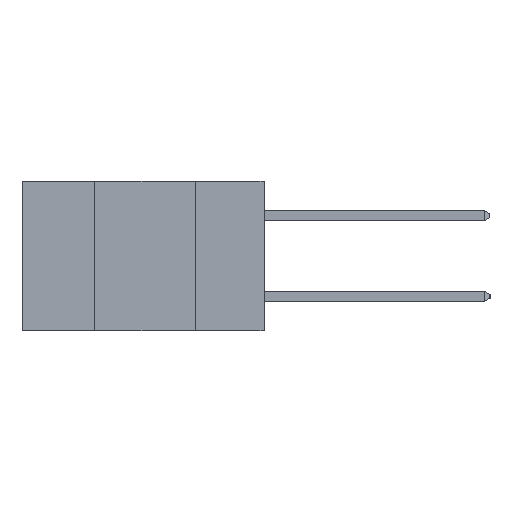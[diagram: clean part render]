
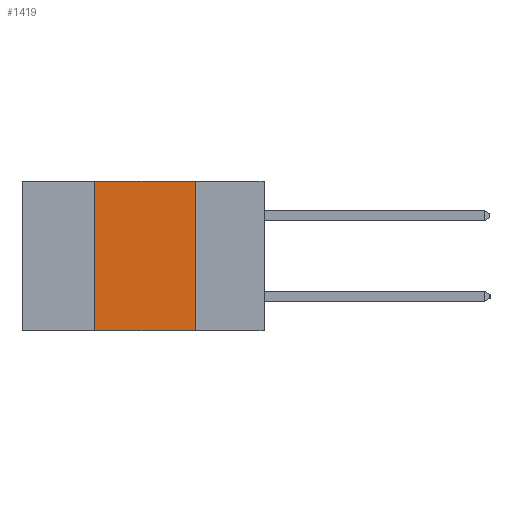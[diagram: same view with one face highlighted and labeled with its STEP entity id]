
A CAD part, left-side view. The second image highlights one B-rep face of the part: STEP entity #1419.
In plain terms, the highlighted planar face has unit normal (-1, 0, 0).
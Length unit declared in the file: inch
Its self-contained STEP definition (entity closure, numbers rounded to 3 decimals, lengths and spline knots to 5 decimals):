
#192 = FACE_OUTER_BOUND ( 'NONE', #4819, .T. ) ;
#352 = CARTESIAN_POINT ( 'NONE',  ( 0., 0.6, 0. ) ) ;
#480 = CARTESIAN_POINT ( 'NONE',  ( 0., 0.17, -0.37 ) ) ;
#930 = CARTESIAN_POINT ( 'NONE',  ( 0., 0.42, 0. ) ) ;
#1086 = CARTESIAN_POINT ( 'NONE',  ( 0., 0.17, -0.37 ) ) ;
#1196 = DIRECTION ( 'NONE',  ( 0., 0., 1. ) ) ;
#1291 = CARTESIAN_POINT ( 'NONE',  ( 0., 0.6, 0. ) ) ;
#1419 = ADVANCED_FACE ( 'NONE', ( #192 ), #9991, .F. ) ;
#1448 = VERTEX_POINT ( 'NONE', #480 ) ;
#1809 = AXIS2_PLACEMENT_3D ( 'NONE', #1291, #6893, #2148 ) ;
#1922 = EDGE_CURVE ( 'NONE', #8537, #1448, #5572, .T. ) ;
#1988 = EDGE_CURVE ( 'NONE', #4662, #8537, #4580, .T. ) ;
#2014 = EDGE_CURVE ( 'NONE', #8920, #4662, #6414, .T. ) ;
#2148 = DIRECTION ( 'NONE',  ( 0., 0., -1. ) ) ;
#2177 = EDGE_CURVE ( 'NONE', #8920, #1448, #7286, .T. ) ;
#3690 = DIRECTION ( 'NONE',  ( 0., -1., 0. ) ) ;
#4580 = LINE ( 'NONE', #352, #8494 ) ;
#4662 = VERTEX_POINT ( 'NONE', #930 ) ;
#4819 = EDGE_LOOP ( 'NONE', ( #5735, #5742, #5782, #5834 ) ) ;
#5572 = LINE ( 'NONE', #1086, #7665 ) ;
#5735 = ORIENTED_EDGE ( 'NONE', *, *, #1922, .F. ) ;
#5742 = ORIENTED_EDGE ( 'NONE', *, *, #1988, .F. ) ;
#5782 = ORIENTED_EDGE ( 'NONE', *, *, #2014, .F. ) ;
#5834 = ORIENTED_EDGE ( 'NONE', *, *, #2177, .T. ) ;
#6119 = CARTESIAN_POINT ( 'NONE',  ( 0., 0.42, -0.37 ) ) ;
#6414 = LINE ( 'NONE', #8366, #10317 ) ;
#6696 = DIRECTION ( 'NONE',  ( 0., 0., -1. ) ) ;
#6893 = DIRECTION ( 'NONE',  ( 1., 0., 0. ) ) ;
#7033 = VECTOR ( 'NONE', #8598, 39.37008 ) ;
#7286 = LINE ( 'NONE', #7833, #7033 ) ;
#7665 = VECTOR ( 'NONE', #6696, 39.37008 ) ;
#7833 = CARTESIAN_POINT ( 'NONE',  ( 0., 0.6, -0.37 ) ) ;
#8366 = CARTESIAN_POINT ( 'NONE',  ( 0., 0.42, -0.37 ) ) ;
#8494 = VECTOR ( 'NONE', #3690, 39.37008 ) ;
#8537 = VERTEX_POINT ( 'NONE', #8800 ) ;
#8598 = DIRECTION ( 'NONE',  ( 0., -1., 0. ) ) ;
#8800 = CARTESIAN_POINT ( 'NONE',  ( 0., 0.17, 0. ) ) ;
#8920 = VERTEX_POINT ( 'NONE', #6119 ) ;
#9991 = PLANE ( 'NONE',  #1809 ) ;
#10317 = VECTOR ( 'NONE', #1196, 39.37008 ) ;
